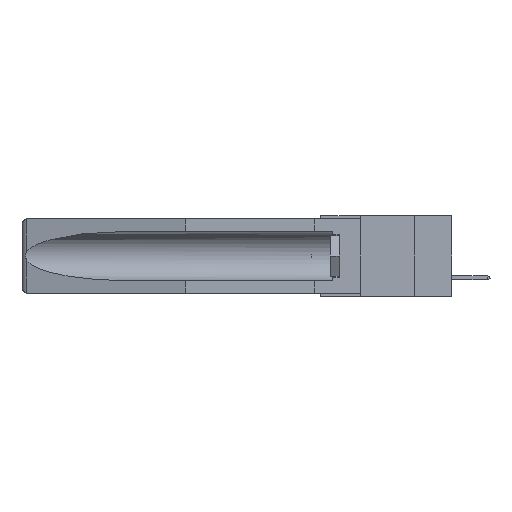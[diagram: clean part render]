
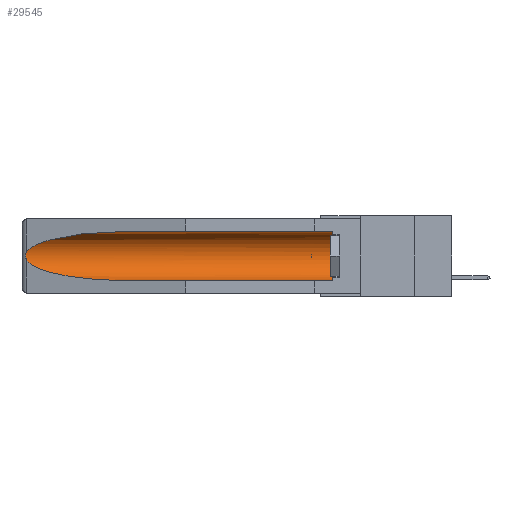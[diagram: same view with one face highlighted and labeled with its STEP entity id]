
A CAD part, left-side view. The second image highlights one B-rep face of the part: STEP entity #29545.
In plain terms, the highlighted cylindrical face has radius 2.857 mm (diameter 5.715 mm), a partial arc.
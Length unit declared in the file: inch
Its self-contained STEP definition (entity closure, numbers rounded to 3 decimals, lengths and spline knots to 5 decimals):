
#12 = CARTESIAN_POINT ( 'NONE',  ( 0.2675, 1.53308, -0.17534 ) ) ;
#894 = LINE ( 'NONE', #17265, #1274 ) ;
#1274 = VECTOR ( 'NONE', #33246, 39.37008 ) ;
#1300 = CIRCLE ( 'NONE', #22301, 0.1125 ) ;
#3623 = EDGE_CURVE ( 'NONE', #13364, #22228, #16877, .T. ) ;
#4118 = ORIENTED_EDGE ( 'NONE', *, *, #3623, .T. ) ;
#4285 = VECTOR ( 'NONE', #31612, 39.37008 ) ;
#4473 = CARTESIAN_POINT ( 'NONE',  ( 0.155, 1.07973, -0.059 ) ) ;
#4550 = VERTEX_POINT ( 'NONE', #34154 ) ;
#4730 = EDGE_CURVE ( 'NONE', #4550, #17504, #6063, .T. ) ;
#4836 = EDGE_CURVE ( 'NONE', #32174, #13364, #1300, .T. ) ;
#5457 = CARTESIAN_POINT ( 'NONE',  ( 0.26655, 1.53094, -0.18657 ) ) ;
#5766 = EDGE_CURVE ( 'NONE', #17504, #18084, #34011, .T. ) ;
#6063 = B_SPLINE_CURVE_WITH_KNOTS ( 'NONE', 3,
 ( #21012, #21476, #26466, #31751, #10408, #12, #29011, #5457, #18566, #13447 ),
 .UNSPECIFIED., .F., .F.,
 ( 4, 2, 2, 2, 4 ),
 ( 0., 0.00029, 0.00058, 0.00087, 0.00117 ),
 .UNSPECIFIED. ) ;
#8222 = CARTESIAN_POINT ( 'NONE',  ( 0.155, 1.07973, -0.059 ) ) ;
#8518 = FACE_OUTER_BOUND ( 'NONE', #10041, .T. ) ;
#9395 = DIRECTION ( 'NONE',  ( 0., 1., 0. ) ) ;
#10041 = EDGE_LOOP ( 'NONE', ( #10765, #25505, #21978, #22715, #31759, #4118 ) ) ;
#10408 = CARTESIAN_POINT ( 'NONE',  ( 0.2675, 1.53308, -0.16763 ) ) ;
#10707 = CARTESIAN_POINT ( 'NONE',  ( 0.26537, 1.52718, -0.19328 ) ) ;
#10765 = ORIENTED_EDGE ( 'NONE', *, *, #15574, .T. ) ;
#10944 = CARTESIAN_POINT ( 'NONE',  ( 0.21114, 1.30732, -0.059 ) ) ;
#12448 = DIRECTION ( 'NONE',  ( 0., 0., 1. ) ) ;
#13364 = VERTEX_POINT ( 'NONE', #27241 ) ;
#13447 = CARTESIAN_POINT ( 'NONE',  ( 0.26537, 1.52718, -0.19328 ) ) ;
#14859 = CARTESIAN_POINT ( 'NONE',  ( 0.26537, 1.52718, -0.19328 ) ) ;
#15574 = EDGE_CURVE ( 'NONE', #22228, #4550, #21067, .T. ) ;
#16225 = CARTESIAN_POINT ( 'NONE',  ( 0.155, -0.30754, -0.1715 ) ) ;
#16551 = CARTESIAN_POINT ( 'NONE',  ( 0.155, 0.126, -0.284 ) ) ;
#16877 = LINE ( 'NONE', #33847, #4285 ) ;
#17265 = CARTESIAN_POINT ( 'NONE',  ( 0.155, -0.30754, -0.284 ) ) ;
#17504 = VERTEX_POINT ( 'NONE', #14859 ) ;
#18084 = VERTEX_POINT ( 'NONE', #27126 ) ;
#18566 = CARTESIAN_POINT ( 'NONE',  ( 0.26597, 1.5296, -0.19026 ) ) ;
#19480 = DIRECTION ( 'NONE',  ( 0., -1., 0. ) ) ;
#21012 = CARTESIAN_POINT ( 'NONE',  ( 0.26537, 1.52718, -0.14972 ) ) ;
#21067 =( BOUNDED_CURVE ( )  B_SPLINE_CURVE ( 3, ( #8222, #10944, #23866, #26754 ),
 .UNSPECIFIED., .F., .F. ) 
 B_SPLINE_CURVE_WITH_KNOTS ( ( 4, 4 ),
 ( 4.71239, 6.08839 ),
 .UNSPECIFIED. ) 
 CURVE ( )  GEOMETRIC_REPRESENTATION_ITEM ( )  RATIONAL_B_SPLINE_CURVE ( ( 1., 0.848, 0.848, 1. ) ) 
 REPRESENTATION_ITEM ( '' )  );
#21388 = CARTESIAN_POINT ( 'NONE',  ( 0.25451, 1.48313, -0.24835 ) ) ;
#21476 = CARTESIAN_POINT ( 'NONE',  ( 0.26597, 1.52961, -0.15275 ) ) ;
#21978 = ORIENTED_EDGE ( 'NONE', *, *, #5766, .T. ) ;
#22228 = VERTEX_POINT ( 'NONE', #4473 ) ;
#22301 = AXIS2_PLACEMENT_3D ( 'NONE', #27944, #19480, #27726 ) ;
#22715 = ORIENTED_EDGE ( 'NONE', *, *, #25387, .F. ) ;
#23866 = CARTESIAN_POINT ( 'NONE',  ( 0.25451, 1.48313, -0.09465 ) ) ;
#25387 = EDGE_CURVE ( 'NONE', #32174, #18084, #894, .T. ) ;
#25505 = ORIENTED_EDGE ( 'NONE', *, *, #4730, .T. ) ;
#26466 = CARTESIAN_POINT ( 'NONE',  ( 0.26654, 1.53092, -0.15636 ) ) ;
#26754 = CARTESIAN_POINT ( 'NONE',  ( 0.26537, 1.52718, -0.14972 ) ) ;
#27072 = CARTESIAN_POINT ( 'NONE',  ( 0.21114, 1.30732, -0.284 ) ) ;
#27126 = CARTESIAN_POINT ( 'NONE',  ( 0.155, 1.07973, -0.284 ) ) ;
#27241 = CARTESIAN_POINT ( 'NONE',  ( 0.155, 0.126, -0.059 ) ) ;
#27726 = DIRECTION ( 'NONE',  ( 0., 0., 1. ) ) ;
#27944 = CARTESIAN_POINT ( 'NONE',  ( 0.155, 0.126, -0.1715 ) ) ;
#28841 = CYLINDRICAL_SURFACE ( 'NONE', #29149, 0.1125 ) ;
#29011 = CARTESIAN_POINT ( 'NONE',  ( 0.2673, 1.53269, -0.17917 ) ) ;
#29149 = AXIS2_PLACEMENT_3D ( 'NONE', #16225, #9395, #12448 ) ;
#29385 = CARTESIAN_POINT ( 'NONE',  ( 0.155, 1.07973, -0.284 ) ) ;
#29545 = ADVANCED_FACE ( 'NONE', ( #8518 ), #28841, .F. ) ;
#31612 = DIRECTION ( 'NONE',  ( 0., 1., 0. ) ) ;
#31751 = CARTESIAN_POINT ( 'NONE',  ( 0.2673, 1.5327, -0.16383 ) ) ;
#31759 = ORIENTED_EDGE ( 'NONE', *, *, #4836, .T. ) ;
#32174 = VERTEX_POINT ( 'NONE', #16551 ) ;
#33246 = DIRECTION ( 'NONE',  ( 0., 1., 0. ) ) ;
#33847 = CARTESIAN_POINT ( 'NONE',  ( 0.155, -0.30754, -0.059 ) ) ;
#34011 =( BOUNDED_CURVE ( )  B_SPLINE_CURVE ( 3, ( #10707, #21388, #27072, #29385 ),
 .UNSPECIFIED., .F., .F. ) 
 B_SPLINE_CURVE_WITH_KNOTS ( ( 4, 4 ),
 ( 0.1948, 1.5708 ),
 .UNSPECIFIED. ) 
 CURVE ( )  GEOMETRIC_REPRESENTATION_ITEM ( )  RATIONAL_B_SPLINE_CURVE ( ( 1., 0.848, 0.848, 1. ) ) 
 REPRESENTATION_ITEM ( '' )  );
#34154 = CARTESIAN_POINT ( 'NONE',  ( 0.26537, 1.52718, -0.14972 ) ) ;
